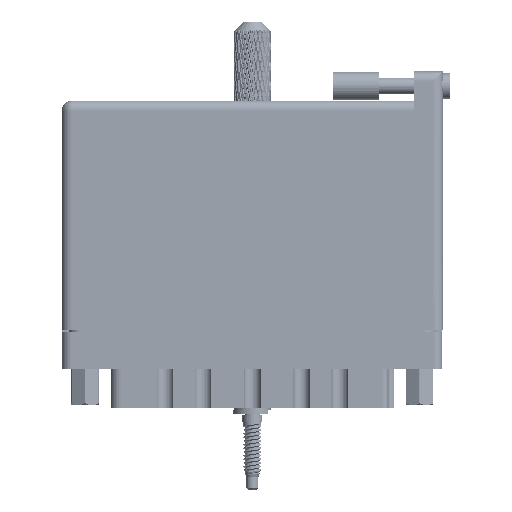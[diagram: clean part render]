
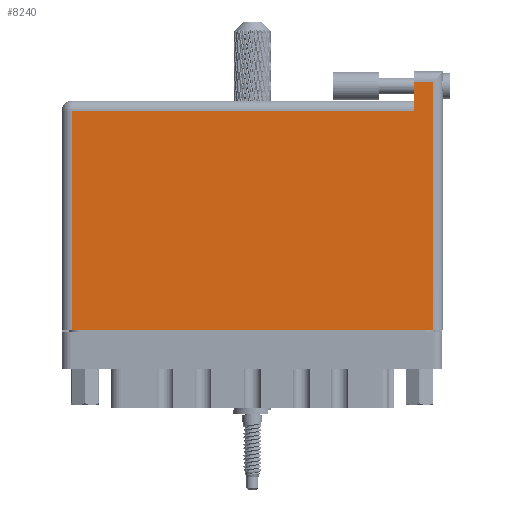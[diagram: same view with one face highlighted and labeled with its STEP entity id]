
A CAD part, front view. The second image highlights one B-rep face of the part: STEP entity #8240.
In plain terms, the highlighted face is planar.
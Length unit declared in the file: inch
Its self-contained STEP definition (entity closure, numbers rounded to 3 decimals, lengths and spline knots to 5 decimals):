
#6092 = VERTEX_POINT ( 'NONE', #88532 ) ;
#8240 = ADVANCED_FACE ( 'NONE', ( #100355 ), #28651, .F. ) ;
#9094 = ORIENTED_EDGE ( 'NONE', *, *, #102214, .T. ) ;
#9647 = DIRECTION ( 'NONE',  ( 0., -1., 0. ) ) ;
#12401 = ORIENTED_EDGE ( 'NONE', *, *, #49139, .T. ) ;
#13666 = DIRECTION ( 'NONE',  ( -1., 0., 0. ) ) ;
#22662 = DIRECTION ( 'NONE',  ( 0., -1., 0. ) ) ;
#28599 = CARTESIAN_POINT ( 'NONE',  ( 0.07, 0., 0. ) ) ;
#28651 = PLANE ( 'NONE',  #68461 ) ;
#32210 = CARTESIAN_POINT ( 'NONE',  ( 2.53, 1.766, 0. ) ) ;
#33580 = DIRECTION ( 'NONE',  ( -1., 0., 0. ) ) ;
#35201 = VECTOR ( 'NONE', #22662, 39.37008 ) ;
#37298 = EDGE_CURVE ( 'NONE', #58498, #119358, #39637, .T. ) ;
#38588 = CARTESIAN_POINT ( 'NONE',  ( 0., 0., 0. ) ) ;
#39637 = LINE ( 'NONE', #38588, #90722 ) ;
#39715 = CARTESIAN_POINT ( 'NONE',  ( 2.403, 1.766, 0. ) ) ;
#40672 = LINE ( 'NONE', #113346, #87204 ) ;
#41764 = ORIENTED_EDGE ( 'NONE', *, *, #37298, .T. ) ;
#43442 = VECTOR ( 'NONE', #122503, 39.37008 ) ;
#49139 = EDGE_CURVE ( 'NONE', #49322, #6092, #64950, .T. ) ;
#49190 = EDGE_LOOP ( 'NONE', ( #41764, #109308, #9094, #12401, #86952, #83417 ) ) ;
#49322 = VERTEX_POINT ( 'NONE', #62736 ) ;
#53588 = LINE ( 'NONE', #61913, #35201 ) ;
#58498 = VERTEX_POINT ( 'NONE', #28599 ) ;
#58884 = VERTEX_POINT ( 'NONE', #90735 ) ;
#61913 = CARTESIAN_POINT ( 'NONE',  ( 0.07, 0., 0. ) ) ;
#62736 = CARTESIAN_POINT ( 'NONE',  ( 2.403, 1.696, 0. ) ) ;
#63359 = CARTESIAN_POINT ( 'NONE',  ( 0., 1.696, 0. ) ) ;
#64950 = LINE ( 'NONE', #39715, #91359 ) ;
#66553 = EDGE_CURVE ( 'NONE', #119358, #122370, #71281, .T. ) ;
#68461 = AXIS2_PLACEMENT_3D ( 'NONE', #127167, #107713, #117220 ) ;
#71281 = LINE ( 'NONE', #32210, #43442 ) ;
#75557 = CARTESIAN_POINT ( 'NONE',  ( 2.53, 1.696, 0. ) ) ;
#83417 = ORIENTED_EDGE ( 'NONE', *, *, #101407, .T. ) ;
#86952 = ORIENTED_EDGE ( 'NONE', *, *, #119265, .T. ) ;
#87204 = VECTOR ( 'NONE', #13666, 39.37008 ) ;
#88532 = CARTESIAN_POINT ( 'NONE',  ( 2.403, 1.496, 0. ) ) ;
#90722 = VECTOR ( 'NONE', #107745, 39.37008 ) ;
#90735 = CARTESIAN_POINT ( 'NONE',  ( 0.07, 1.496, 0. ) ) ;
#91359 = VECTOR ( 'NONE', #9647, 39.37008 ) ;
#100355 = FACE_OUTER_BOUND ( 'NONE', #49190, .T. ) ;
#101407 = EDGE_CURVE ( 'NONE', #58884, #58498, #53588, .T. ) ;
#102214 = EDGE_CURVE ( 'NONE', #122370, #49322, #106141, .T. ) ;
#106141 = LINE ( 'NONE', #63359, #124583 ) ;
#107713 = DIRECTION ( 'NONE',  ( 0., 0., -1. ) ) ;
#107745 = DIRECTION ( 'NONE',  ( 1., 0., 0. ) ) ;
#109308 = ORIENTED_EDGE ( 'NONE', *, *, #66553, .T. ) ;
#111626 = CARTESIAN_POINT ( 'NONE',  ( 2.53, 0., 0. ) ) ;
#113346 = CARTESIAN_POINT ( 'NONE',  ( 0., 1.496, 0. ) ) ;
#117220 = DIRECTION ( 'NONE',  ( -1., 0., 0. ) ) ;
#119265 = EDGE_CURVE ( 'NONE', #6092, #58884, #40672, .T. ) ;
#119358 = VERTEX_POINT ( 'NONE', #111626 ) ;
#122370 = VERTEX_POINT ( 'NONE', #75557 ) ;
#122503 = DIRECTION ( 'NONE',  ( 0., 1., 0. ) ) ;
#124583 = VECTOR ( 'NONE', #33580, 39.37008 ) ;
#127167 = CARTESIAN_POINT ( 'NONE',  ( 0., 1.566, 0. ) ) ;
